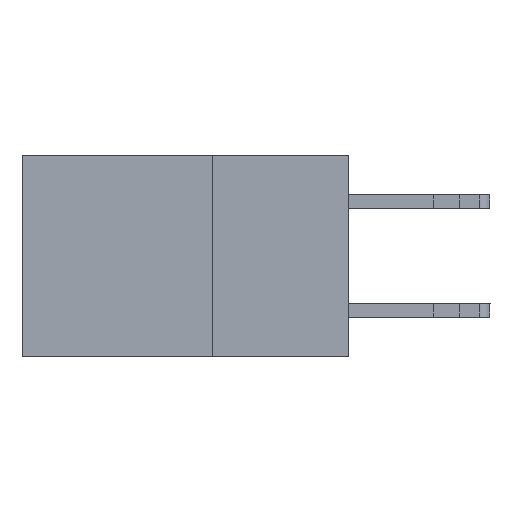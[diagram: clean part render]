
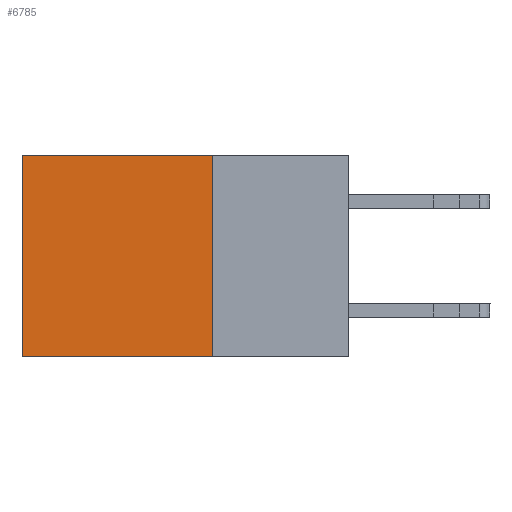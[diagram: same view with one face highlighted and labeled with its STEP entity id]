
A CAD part, left-side view. The second image highlights one B-rep face of the part: STEP entity #6785.
In plain terms, the highlighted planar face has unit normal (-1, 0, 0).
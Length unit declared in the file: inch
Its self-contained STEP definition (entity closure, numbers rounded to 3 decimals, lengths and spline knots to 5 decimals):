
#762 = CARTESIAN_POINT ( 'NONE',  ( 0.2615, 0.6, 0. ) ) ;
#838 = DIRECTION ( 'NONE',  ( 0., 0., -1. ) ) ;
#1113 = AXIS2_PLACEMENT_3D ( 'NONE', #6944, #6732, #6688 ) ;
#1187 = ORIENTED_EDGE ( 'NONE', *, *, #13002, .T. ) ;
#1229 = LINE ( 'NONE', #6390, #12149 ) ;
#1862 = EDGE_CURVE ( 'NONE', #9613, #2845, #4332, .T. ) ;
#2272 = CARTESIAN_POINT ( 'NONE',  ( 0.2615, 0.25, -0.37 ) ) ;
#2394 = DIRECTION ( 'NONE',  ( 0., 0., -1. ) ) ;
#2845 = VERTEX_POINT ( 'NONE', #8360 ) ;
#3166 = VECTOR ( 'NONE', #12747, 39.37008 ) ;
#3446 = EDGE_CURVE ( 'NONE', #11591, #12170, #3881, .T. ) ;
#3881 = LINE ( 'NONE', #12855, #3166 ) ;
#4155 = EDGE_LOOP ( 'NONE', ( #1187, #13272, #9206, #12727 ) ) ;
#4332 = LINE ( 'NONE', #13537, #9931 ) ;
#4609 = CARTESIAN_POINT ( 'NONE',  ( 0.2615, 0.25, 0. ) ) ;
#5399 = LINE ( 'NONE', #2272, #9949 ) ;
#5580 = FACE_OUTER_BOUND ( 'NONE', #4155, .T. ) ;
#6390 = CARTESIAN_POINT ( 'NONE',  ( 0.2615, 0.6, -0.37 ) ) ;
#6688 = DIRECTION ( 'NONE',  ( 0., 0., -1. ) ) ;
#6732 = DIRECTION ( 'NONE',  ( 1., 0., 0. ) ) ;
#6785 = ADVANCED_FACE ( 'NONE', ( #5580 ), #7179, .F. ) ;
#6944 = CARTESIAN_POINT ( 'NONE',  ( 0.2615, 0.25, -0.37 ) ) ;
#7057 = EDGE_CURVE ( 'NONE', #11591, #9613, #5399, .T. ) ;
#7179 = PLANE ( 'NONE',  #1113 ) ;
#8360 = CARTESIAN_POINT ( 'NONE',  ( 0.2615, 0.6, -0.37 ) ) ;
#9206 = ORIENTED_EDGE ( 'NONE', *, *, #7057, .F. ) ;
#9613 = VERTEX_POINT ( 'NONE', #13184 ) ;
#9931 = VECTOR ( 'NONE', #13195, 39.37008 ) ;
#9949 = VECTOR ( 'NONE', #2394, 39.37008 ) ;
#11591 = VERTEX_POINT ( 'NONE', #4609 ) ;
#12149 = VECTOR ( 'NONE', #838, 39.37008 ) ;
#12170 = VERTEX_POINT ( 'NONE', #762 ) ;
#12727 = ORIENTED_EDGE ( 'NONE', *, *, #3446, .T. ) ;
#12747 = DIRECTION ( 'NONE',  ( 0., 1., 0. ) ) ;
#12855 = CARTESIAN_POINT ( 'NONE',  ( 0.2615, 0.25, 0. ) ) ;
#13002 = EDGE_CURVE ( 'NONE', #12170, #2845, #1229, .T. ) ;
#13184 = CARTESIAN_POINT ( 'NONE',  ( 0.2615, 0.25, -0.37 ) ) ;
#13195 = DIRECTION ( 'NONE',  ( 0., 1., 0. ) ) ;
#13272 = ORIENTED_EDGE ( 'NONE', *, *, #1862, .F. ) ;
#13537 = CARTESIAN_POINT ( 'NONE',  ( 0.2615, 0.25, -0.37 ) ) ;
